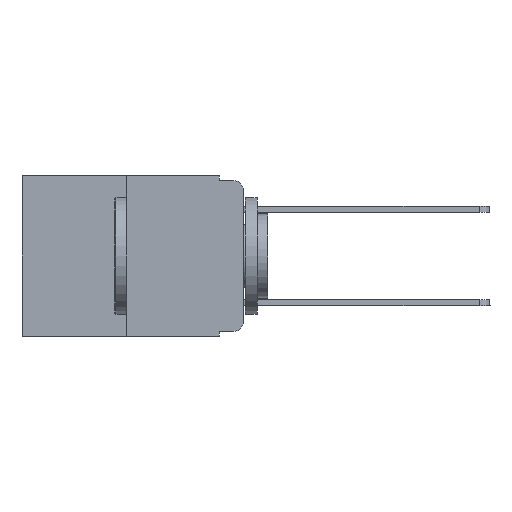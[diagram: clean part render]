
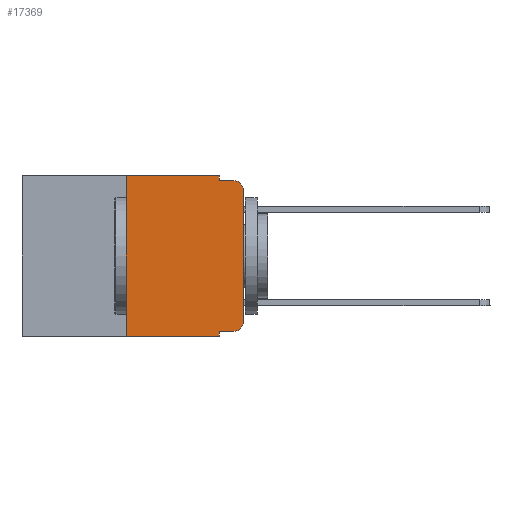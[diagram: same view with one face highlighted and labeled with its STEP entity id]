
A CAD part, left-side view. The second image highlights one B-rep face of the part: STEP entity #17369.
In plain terms, the highlighted planar face has unit normal (-1, 0, 0).
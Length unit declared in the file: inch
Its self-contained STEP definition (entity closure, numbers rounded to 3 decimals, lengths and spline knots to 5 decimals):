
#216 = DIRECTION ( 'NONE',  ( 0., 0., -1. ) ) ;
#888 = ORIENTED_EDGE ( 'NONE', *, *, #10510, .T. ) ;
#910 = VECTOR ( 'NONE', #5537, 39.37008 ) ;
#1348 = EDGE_CURVE ( 'NONE', #19319, #14699, #15744, .T. ) ;
#1364 = CARTESIAN_POINT ( 'NONE',  ( 0., 0.051, -0.343 ) ) ;
#1763 = ORIENTED_EDGE ( 'NONE', *, *, #6379, .T. ) ;
#1839 = VECTOR ( 'NONE', #18231, 39.37008 ) ;
#1998 = EDGE_CURVE ( 'NONE', #21155, #10043, #5074, .T. ) ;
#2160 = ORIENTED_EDGE ( 'NONE', *, *, #6110, .F. ) ;
#2282 = CARTESIAN_POINT ( 'NONE',  ( 0., 0.02, -0.333 ) ) ;
#2498 = EDGE_CURVE ( 'NONE', #14013, #9781, #10367, .T. ) ;
#3225 = ORIENTED_EDGE ( 'NONE', *, *, #3961, .F. ) ;
#3419 = CARTESIAN_POINT ( 'NONE',  ( 0., 0., 0. ) ) ;
#3961 = EDGE_CURVE ( 'NONE', #19319, #9873, #9186, .T. ) ;
#3983 = AXIS2_PLACEMENT_3D ( 'NONE', #19351, #11097, #14560 ) ;
#4347 = ORIENTED_EDGE ( 'NONE', *, *, #1998, .F. ) ;
#4582 = CIRCLE ( 'NONE', #19176, 0.02 ) ;
#4587 = CARTESIAN_POINT ( 'NONE',  ( 0., 0.051, 0. ) ) ;
#4691 = CIRCLE ( 'NONE', #3983, 0.02 ) ;
#5074 = LINE ( 'NONE', #5172, #5605 ) ;
#5172 = CARTESIAN_POINT ( 'NONE',  ( 0., 0.051, -0.01 ) ) ;
#5490 = CARTESIAN_POINT ( 'NONE',  ( 0., 0.051, -0.333 ) ) ;
#5537 = DIRECTION ( 'NONE',  ( 0., -1., 0. ) ) ;
#5605 = VECTOR ( 'NONE', #8649, 39.37008 ) ;
#6110 = EDGE_CURVE ( 'NONE', #14940, #14699, #11774, .T. ) ;
#6379 = EDGE_CURVE ( 'NONE', #15812, #14013, #4691, .T. ) ;
#6425 = VECTOR ( 'NONE', #10026, 39.37008 ) ;
#7206 = VERTEX_POINT ( 'NONE', #4587 ) ;
#7674 = FACE_OUTER_BOUND ( 'NONE', #13152, .T. ) ;
#8649 = DIRECTION ( 'NONE',  ( 0., -1., 0. ) ) ;
#8801 = LINE ( 'NONE', #14025, #910 ) ;
#9068 = CARTESIAN_POINT ( 'NONE',  ( 0., 0.25, 0. ) ) ;
#9186 = LINE ( 'NONE', #9068, #16345 ) ;
#9781 = VERTEX_POINT ( 'NONE', #18759 ) ;
#9873 = VERTEX_POINT ( 'NONE', #12890 ) ;
#10026 = DIRECTION ( 'NONE',  ( 0., -1., 0. ) ) ;
#10043 = VERTEX_POINT ( 'NONE', #19953 ) ;
#10063 = DIRECTION ( 'NONE',  ( -1., 0., 0. ) ) ;
#10137 = CARTESIAN_POINT ( 'NONE',  ( 0., 0.051, -0.01 ) ) ;
#10367 = LINE ( 'NONE', #3419, #1839 ) ;
#10510 = EDGE_CURVE ( 'NONE', #14940, #15812, #13287, .T. ) ;
#10789 = VECTOR ( 'NONE', #216, 39.37008 ) ;
#11097 = DIRECTION ( 'NONE',  ( -1., 0., 0. ) ) ;
#11103 = DIRECTION ( 'NONE',  ( 0., -1., 0. ) ) ;
#11354 = ORIENTED_EDGE ( 'NONE', *, *, #1348, .T. ) ;
#11773 = CARTESIAN_POINT ( 'NONE',  ( 0., 0.051, -0.333 ) ) ;
#11774 = LINE ( 'NONE', #18400, #10789 ) ;
#11916 = LINE ( 'NONE', #12228, #16344 ) ;
#12222 = EDGE_CURVE ( 'NONE', #9873, #7206, #8801, .T. ) ;
#12228 = CARTESIAN_POINT ( 'NONE',  ( 0., 0.051, 0. ) ) ;
#12703 = CARTESIAN_POINT ( 'NONE',  ( 0., 0.473, 0. ) ) ;
#12890 = CARTESIAN_POINT ( 'NONE',  ( 0., 0.25, 0. ) ) ;
#13152 = EDGE_LOOP ( 'NONE', ( #18561, #19480, #4347, #18154, #16889, #3225, #11354, #2160, #888, #1763 ) ) ;
#13287 = LINE ( 'NONE', #11773, #6425 ) ;
#13561 = AXIS2_PLACEMENT_3D ( 'NONE', #12703, #20879, #19333 ) ;
#14013 = VERTEX_POINT ( 'NONE', #15237 ) ;
#14025 = CARTESIAN_POINT ( 'NONE',  ( 0., 0.473, 0. ) ) ;
#14560 = DIRECTION ( 'NONE',  ( 0., 0., -1. ) ) ;
#14699 = VERTEX_POINT ( 'NONE', #1364 ) ;
#14940 = VERTEX_POINT ( 'NONE', #5490 ) ;
#15041 = CARTESIAN_POINT ( 'NONE',  ( 0., 0.02, -0.03 ) ) ;
#15237 = CARTESIAN_POINT ( 'NONE',  ( 0., 0., -0.313 ) ) ;
#15577 = DIRECTION ( 'NONE',  ( 0., 0., 1. ) ) ;
#15744 = LINE ( 'NONE', #17406, #15930 ) ;
#15812 = VERTEX_POINT ( 'NONE', #2282 ) ;
#15930 = VECTOR ( 'NONE', #11103, 39.37008 ) ;
#15938 = PLANE ( 'NONE',  #13561 ) ;
#16344 = VECTOR ( 'NONE', #17223, 39.37008 ) ;
#16345 = VECTOR ( 'NONE', #15577, 39.37008 ) ;
#16889 = ORIENTED_EDGE ( 'NONE', *, *, #12222, .F. ) ;
#16908 = DIRECTION ( 'NONE',  ( 0., 0., -1. ) ) ;
#17223 = DIRECTION ( 'NONE',  ( 0., 0., -1. ) ) ;
#17369 = ADVANCED_FACE ( 'NONE', ( #7674 ), #15938, .F. ) ;
#17406 = CARTESIAN_POINT ( 'NONE',  ( 0., 0.473, -0.343 ) ) ;
#18078 = EDGE_CURVE ( 'NONE', #7206, #21155, #11916, .T. ) ;
#18154 = ORIENTED_EDGE ( 'NONE', *, *, #18078, .F. ) ;
#18231 = DIRECTION ( 'NONE',  ( 0., 0., 1. ) ) ;
#18400 = CARTESIAN_POINT ( 'NONE',  ( 0., 0.051, 0. ) ) ;
#18561 = ORIENTED_EDGE ( 'NONE', *, *, #2498, .T. ) ;
#18759 = CARTESIAN_POINT ( 'NONE',  ( 0., 0., -0.03 ) ) ;
#19176 = AXIS2_PLACEMENT_3D ( 'NONE', #15041, #10063, #16908 ) ;
#19294 = EDGE_CURVE ( 'NONE', #9781, #10043, #4582, .T. ) ;
#19319 = VERTEX_POINT ( 'NONE', #19847 ) ;
#19333 = DIRECTION ( 'NONE',  ( 0., 0., -1. ) ) ;
#19351 = CARTESIAN_POINT ( 'NONE',  ( 0., 0.02, -0.313 ) ) ;
#19480 = ORIENTED_EDGE ( 'NONE', *, *, #19294, .T. ) ;
#19847 = CARTESIAN_POINT ( 'NONE',  ( 0., 0.25, -0.343 ) ) ;
#19953 = CARTESIAN_POINT ( 'NONE',  ( 0., 0.02, -0.01 ) ) ;
#20879 = DIRECTION ( 'NONE',  ( 1., 0., 0. ) ) ;
#21155 = VERTEX_POINT ( 'NONE', #10137 ) ;
